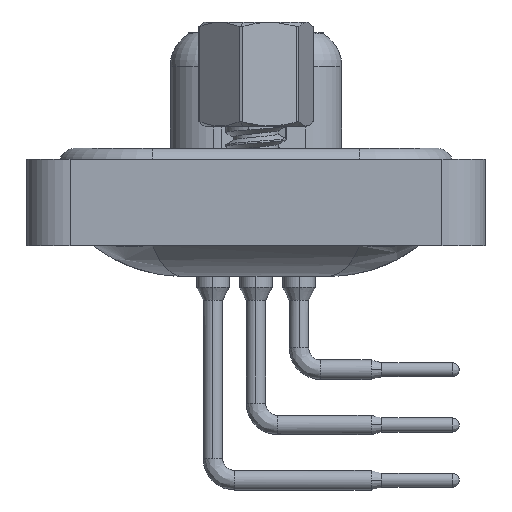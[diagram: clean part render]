
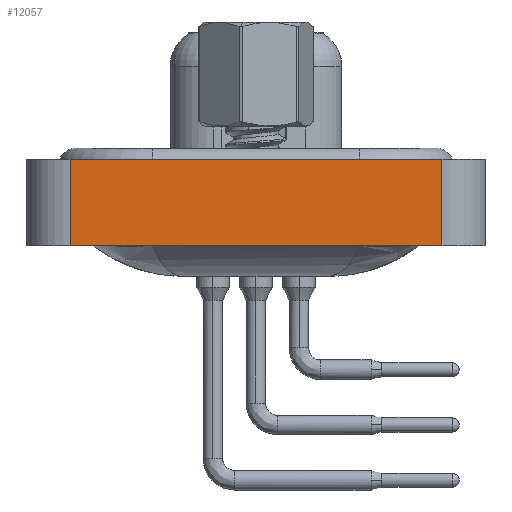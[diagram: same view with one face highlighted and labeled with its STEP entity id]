
A CAD part, left-side view. The second image highlights one B-rep face of the part: STEP entity #12057.
In plain terms, the highlighted planar face has unit normal (-1, 0, 0).
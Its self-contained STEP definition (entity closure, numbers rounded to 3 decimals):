
#2075 = VECTOR ( 'NONE', #3265, 1000. ) ;
#2402 = EDGE_CURVE ( 'NONE', #11137, #18752, #12264, .T. ) ;
#2842 = EDGE_CURVE ( 'NONE', #18886, #12922, #9614, .T. ) ;
#3265 = DIRECTION ( 'NONE',  ( 0., 0., 1. ) ) ;
#3927 = EDGE_CURVE ( 'NONE', #18752, #12922, #12342, .T. ) ;
#4842 = CARTESIAN_POINT ( 'NONE',  ( -7.35, -8.55, -3.6 ) ) ;
#5624 = EDGE_LOOP ( 'NONE', ( #30769, #14940, #33104, #26258 ) ) ;
#6736 = DIRECTION ( 'NONE',  ( 0., -1., 0. ) ) ;
#9614 = LINE ( 'NONE', #15982, #2075 ) ;
#11137 = VERTEX_POINT ( 'NONE', #14291 ) ;
#12057 = ADVANCED_FACE ( 'NONE', ( #23159 ), #32157, .T. ) ;
#12264 = LINE ( 'NONE', #21830, #34517 ) ;
#12342 = LINE ( 'NONE', #26901, #27612 ) ;
#12922 = VERTEX_POINT ( 'NONE', #29783 ) ;
#14291 = CARTESIAN_POINT ( 'NONE',  ( -7.35, 8.55, -3.6 ) ) ;
#14817 = VECTOR ( 'NONE', #6736, 1000. ) ;
#14940 = ORIENTED_EDGE ( 'NONE', *, *, #3927, .F. ) ;
#15982 = CARTESIAN_POINT ( 'NONE',  ( -7.35, -8.55, -3.6 ) ) ;
#17290 = AXIS2_PLACEMENT_3D ( 'NONE', #4842, #32733, #19988 ) ;
#18752 = VERTEX_POINT ( 'NONE', #28411 ) ;
#18886 = VERTEX_POINT ( 'NONE', #26609 ) ;
#19988 = DIRECTION ( 'NONE',  ( 0., 0., 1. ) ) ;
#21830 = CARTESIAN_POINT ( 'NONE',  ( -7.35, 8.55, -3.6 ) ) ;
#23159 = FACE_OUTER_BOUND ( 'NONE', #5624, .T. ) ;
#23999 = EDGE_CURVE ( 'NONE', #11137, #18886, #27854, .T. ) ;
#26258 = ORIENTED_EDGE ( 'NONE', *, *, #23999, .T. ) ;
#26609 = CARTESIAN_POINT ( 'NONE',  ( -7.35, -8.55, -3.6 ) ) ;
#26901 = CARTESIAN_POINT ( 'NONE',  ( -7.35, -8.55, 0.4 ) ) ;
#27612 = VECTOR ( 'NONE', #33475, 1000. ) ;
#27854 = LINE ( 'NONE', #33268, #14817 ) ;
#28188 = DIRECTION ( 'NONE',  ( 0., 0., 1. ) ) ;
#28411 = CARTESIAN_POINT ( 'NONE',  ( -7.35, 8.55, 0.4 ) ) ;
#29783 = CARTESIAN_POINT ( 'NONE',  ( -7.35, -8.55, 0.4 ) ) ;
#30769 = ORIENTED_EDGE ( 'NONE', *, *, #2842, .T. ) ;
#32157 = PLANE ( 'NONE',  #17290 ) ;
#32733 = DIRECTION ( 'NONE',  ( -1., 0., 0. ) ) ;
#33104 = ORIENTED_EDGE ( 'NONE', *, *, #2402, .F. ) ;
#33268 = CARTESIAN_POINT ( 'NONE',  ( -7.35, -8.55, -3.6 ) ) ;
#33475 = DIRECTION ( 'NONE',  ( 0., -1., 0. ) ) ;
#34517 = VECTOR ( 'NONE', #28188, 1000. ) ;
